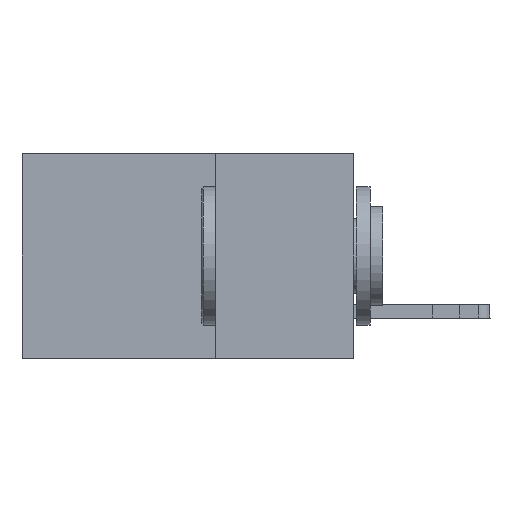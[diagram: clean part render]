
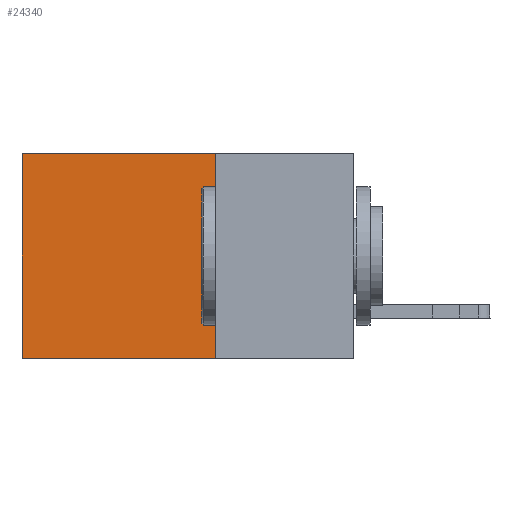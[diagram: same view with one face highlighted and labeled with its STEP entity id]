
A CAD part, left-side view. The second image highlights one B-rep face of the part: STEP entity #24340.
In plain terms, the highlighted planar face has unit normal (-1, 0, 0).
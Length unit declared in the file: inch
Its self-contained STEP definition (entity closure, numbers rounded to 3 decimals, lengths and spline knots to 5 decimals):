
#825 = VERTEX_POINT ( 'NONE', #32435 ) ;
#3064 = VECTOR ( 'NONE', #33172, 39.37008 ) ;
#3271 = VECTOR ( 'NONE', #3843, 39.37008 ) ;
#3843 = DIRECTION ( 'NONE',  ( 0., 1., 0. ) ) ;
#5032 = ORIENTED_EDGE ( 'NONE', *, *, #21470, .F. ) ;
#6353 = VECTOR ( 'NONE', #13799, 39.37008 ) ;
#6539 = CARTESIAN_POINT ( 'NONE',  ( 0.2875, 0.6, 0. ) ) ;
#7052 = LINE ( 'NONE', #30974, #35701 ) ;
#8245 = EDGE_LOOP ( 'NONE', ( #33332, #9014, #5032, #22381 ) ) ;
#9014 = ORIENTED_EDGE ( 'NONE', *, *, #34136, .F. ) ;
#9472 = CARTESIAN_POINT ( 'NONE',  ( 0.2875, 0.25, 0. ) ) ;
#10392 = CARTESIAN_POINT ( 'NONE',  ( 0.2875, 0.25, 0. ) ) ;
#10985 = DIRECTION ( 'NONE',  ( 0., 1., 0. ) ) ;
#11815 = LINE ( 'NONE', #9472, #3271 ) ;
#13271 = DIRECTION ( 'NONE',  ( 1., 0., 0. ) ) ;
#13799 = DIRECTION ( 'NONE',  ( 0., 0., -1. ) ) ;
#14844 = CARTESIAN_POINT ( 'NONE',  ( 0.2875, 0.25, -0.37 ) ) ;
#15843 = CARTESIAN_POINT ( 'NONE',  ( 0.2875, 0.6, -0.37 ) ) ;
#18171 = VERTEX_POINT ( 'NONE', #6539 ) ;
#18742 = FACE_OUTER_BOUND ( 'NONE', #8245, .T. ) ;
#20478 = EDGE_CURVE ( 'NONE', #825, #18171, #11815, .T. ) ;
#21470 = EDGE_CURVE ( 'NONE', #825, #32528, #36781, .T. ) ;
#22381 = ORIENTED_EDGE ( 'NONE', *, *, #20478, .T. ) ;
#23701 = EDGE_CURVE ( 'NONE', #18171, #34604, #34426, .T. ) ;
#24340 = ADVANCED_FACE ( 'NONE', ( #18742 ), #27499, .F. ) ;
#27499 = PLANE ( 'NONE',  #30781 ) ;
#30781 = AXIS2_PLACEMENT_3D ( 'NONE', #10392, #13271, #33254 ) ;
#30909 = CARTESIAN_POINT ( 'NONE',  ( 0.2875, 0.25, 0. ) ) ;
#30974 = CARTESIAN_POINT ( 'NONE',  ( 0.2875, 0.25, -0.37 ) ) ;
#32435 = CARTESIAN_POINT ( 'NONE',  ( 0.2875, 0.25, 0. ) ) ;
#32528 = VERTEX_POINT ( 'NONE', #14844 ) ;
#33172 = DIRECTION ( 'NONE',  ( 0., 0., -1. ) ) ;
#33254 = DIRECTION ( 'NONE',  ( 0., 0., -1. ) ) ;
#33332 = ORIENTED_EDGE ( 'NONE', *, *, #23701, .T. ) ;
#34136 = EDGE_CURVE ( 'NONE', #32528, #34604, #7052, .T. ) ;
#34426 = LINE ( 'NONE', #36067, #3064 ) ;
#34604 = VERTEX_POINT ( 'NONE', #15843 ) ;
#35701 = VECTOR ( 'NONE', #10985, 39.37008 ) ;
#36067 = CARTESIAN_POINT ( 'NONE',  ( 0.2875, 0.6, 0. ) ) ;
#36781 = LINE ( 'NONE', #30909, #6353 ) ;
